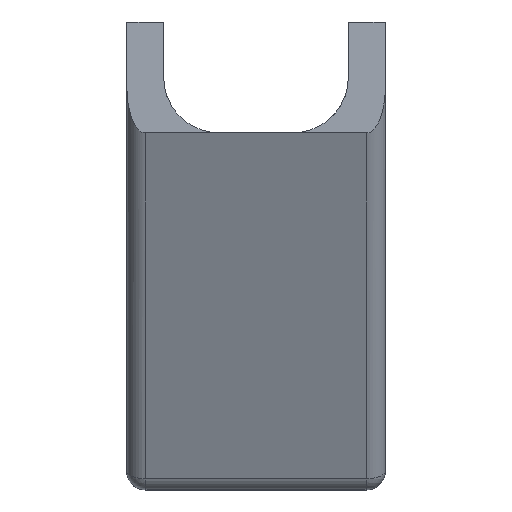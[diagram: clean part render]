
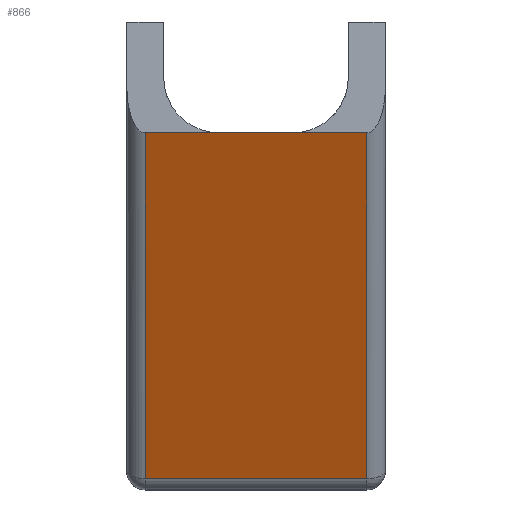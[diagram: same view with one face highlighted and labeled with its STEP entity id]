
A CAD part, top view. The second image highlights one B-rep face of the part: STEP entity #866.
In plain terms, the highlighted planar face has unit normal (0, -0.404, 0.915).
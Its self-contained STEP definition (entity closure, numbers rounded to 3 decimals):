
#3 = CARTESIAN_POINT ( 'NONE',  ( 25., -19.135, 17.761 ) ) ;
#115 = VERTEX_POINT ( 'NONE', #1503 ) ;
#124 = VERTEX_POINT ( 'NONE', #1508 ) ;
#139 = VERTEX_POINT ( 'NONE', #1491 ) ;
#228 = VECTOR ( 'NONE', #1719, 1000. ) ;
#320 = CARTESIAN_POINT ( 'NONE',  ( 10., -19.135, 17.761 ) ) ;
#332 = DIRECTION ( 'NONE',  ( 0., 0.915, 0.404 ) ) ;
#342 = DIRECTION ( 'NONE',  ( 0., 0.404, -0.915 ) ) ;
#419 = CARTESIAN_POINT ( 'NONE',  ( 70., -19.135, 17.761 ) ) ;
#433 = VECTOR ( 'NONE', #1275, 1000. ) ;
#473 = DIRECTION ( 'NONE',  ( 1., 0., 0. ) ) ;
#507 = VERTEX_POINT ( 'NONE', #772 ) ;
#541 = EDGE_LOOP ( 'NONE', ( #1154, #1305, #1360, #1373, #1374, #1398 ) ) ;
#581 = DIRECTION ( 'NONE',  ( -1., 0., 0. ) ) ;
#772 = CARTESIAN_POINT ( 'NONE',  ( 5., -112.689, -23.523 ) ) ;
#832 = VECTOR ( 'NONE', #1296, 1000. ) ;
#860 = VECTOR ( 'NONE', #581, 1000. ) ;
#866 = ADVANCED_FACE ( 'NONE', ( #1634 ), #1020, .F. ) ;
#891 = VECTOR ( 'NONE', #473, 1000. ) ;
#969 = CARTESIAN_POINT ( 'NONE',  ( 70., -112.689, -23.523 ) ) ;
#987 = VERTEX_POINT ( 'NONE', #1121 ) ;
#997 = CARTESIAN_POINT ( 'NONE',  ( 65., -19.135, 17.761 ) ) ;
#1008 = CARTESIAN_POINT ( 'NONE',  ( 70., -19.135, 17.761 ) ) ;
#1019 = EDGE_CURVE ( 'NONE', #1397, #115, #1431, .T. ) ;
#1020 = PLANE ( 'NONE',  #1874 ) ;
#1121 = CARTESIAN_POINT ( 'NONE',  ( 65., -112.689, -23.523 ) ) ;
#1154 = ORIENTED_EDGE ( 'NONE', *, *, #1453, .T. ) ;
#1159 = LINE ( 'NONE', #320, #891 ) ;
#1162 = EDGE_CURVE ( 'NONE', #124, #139, #1587, .T. ) ;
#1275 = DIRECTION ( 'NONE',  ( 1., 0., 0. ) ) ;
#1296 = DIRECTION ( 'NONE',  ( 0., 0.915, 0.404 ) ) ;
#1301 = LINE ( 'NONE', #969, #433 ) ;
#1305 = ORIENTED_EDGE ( 'NONE', *, *, #1464, .T. ) ;
#1360 = ORIENTED_EDGE ( 'NONE', *, *, #1162, .T. ) ;
#1373 = ORIENTED_EDGE ( 'NONE', *, *, #1476, .F. ) ;
#1374 = ORIENTED_EDGE ( 'NONE', *, *, #1019, .T. ) ;
#1397 = VERTEX_POINT ( 'NONE', #3 ) ;
#1398 = ORIENTED_EDGE ( 'NONE', *, *, #1478, .T. ) ;
#1431 = LINE ( 'NONE', #1555, #1812 ) ;
#1433 = LINE ( 'NONE', #1581, #228 ) ;
#1453 = EDGE_CURVE ( 'NONE', #507, #987, #1301, .T. ) ;
#1464 = EDGE_CURVE ( 'NONE', #987, #124, #1517, .T. ) ;
#1476 = EDGE_CURVE ( 'NONE', #1397, #139, #1159, .T. ) ;
#1478 = EDGE_CURVE ( 'NONE', #115, #507, #1433, .T. ) ;
#1491 = CARTESIAN_POINT ( 'NONE',  ( 45., -19.135, 17.761 ) ) ;
#1503 = CARTESIAN_POINT ( 'NONE',  ( 5., -19.135, 17.761 ) ) ;
#1508 = CARTESIAN_POINT ( 'NONE',  ( 65., -19.135, 17.761 ) ) ;
#1517 = LINE ( 'NONE', #997, #832 ) ;
#1555 = CARTESIAN_POINT ( 'NONE',  ( 70., -19.135, 17.761 ) ) ;
#1581 = CARTESIAN_POINT ( 'NONE',  ( 5., -19.135, 17.761 ) ) ;
#1587 = LINE ( 'NONE', #419, #860 ) ;
#1634 = FACE_OUTER_BOUND ( 'NONE', #541, .T. ) ;
#1701 = DIRECTION ( 'NONE',  ( -1., 0., 0. ) ) ;
#1719 = DIRECTION ( 'NONE',  ( 0., -0.915, -0.404 ) ) ;
#1812 = VECTOR ( 'NONE', #1701, 1000. ) ;
#1874 = AXIS2_PLACEMENT_3D ( 'NONE', #1008, #342, #332 ) ;
